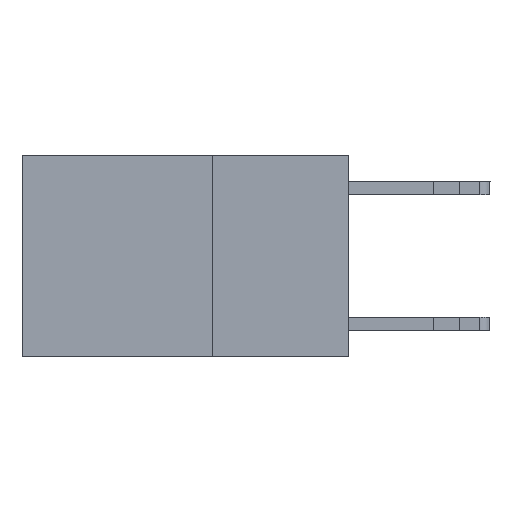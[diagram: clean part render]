
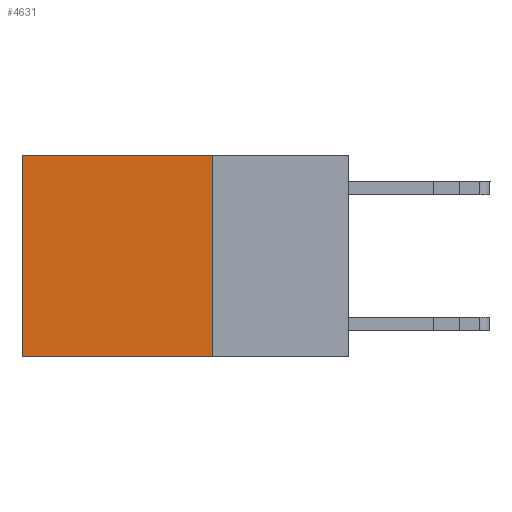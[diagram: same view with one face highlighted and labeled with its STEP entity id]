
A CAD part, left-side view. The second image highlights one B-rep face of the part: STEP entity #4631.
In plain terms, the highlighted planar face has unit normal (-1, 0, 0).
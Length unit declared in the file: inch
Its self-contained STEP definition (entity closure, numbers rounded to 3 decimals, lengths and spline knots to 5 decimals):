
#223 = DIRECTION ( 'NONE',  ( 0., 1., 0. ) ) ;
#496 = DIRECTION ( 'NONE',  ( 0., 1., 0. ) ) ;
#2611 = LINE ( 'NONE', #7251, #3424 ) ;
#2944 = CARTESIAN_POINT ( 'NONE',  ( 0.2625, 0.6, -0.37 ) ) ;
#3009 = ORIENTED_EDGE ( 'NONE', *, *, #6220, .T. ) ;
#3424 = VECTOR ( 'NONE', #496, 39.37008 ) ;
#4271 = DIRECTION ( 'NONE',  ( 1., 0., 0. ) ) ;
#4631 = ADVANCED_FACE ( 'NONE', ( #14182 ), #12147, .F. ) ;
#5284 = EDGE_CURVE ( 'NONE', #7028, #12721, #13727, .T. ) ;
#6003 = EDGE_CURVE ( 'NONE', #12983, #10503, #13409, .T. ) ;
#6211 = CARTESIAN_POINT ( 'NONE',  ( 0.2625, 0.25, 0. ) ) ;
#6220 = EDGE_CURVE ( 'NONE', #7028, #12983, #2611, .T. ) ;
#6309 = ORIENTED_EDGE ( 'NONE', *, *, #7378, .F. ) ;
#6672 = CARTESIAN_POINT ( 'NONE',  ( 0.2625, 0.25, 0. ) ) ;
#6841 = LINE ( 'NONE', #9230, #11049 ) ;
#7028 = VERTEX_POINT ( 'NONE', #9510 ) ;
#7251 = CARTESIAN_POINT ( 'NONE',  ( 0.2625, 0.25, 0. ) ) ;
#7378 = EDGE_CURVE ( 'NONE', #12721, #10503, #6841, .T. ) ;
#7656 = AXIS2_PLACEMENT_3D ( 'NONE', #6672, #4271, #12001 ) ;
#8067 = DIRECTION ( 'NONE',  ( 0., 0., -1. ) ) ;
#8513 = VECTOR ( 'NONE', #8067, 39.37008 ) ;
#8750 = ORIENTED_EDGE ( 'NONE', *, *, #5284, .F. ) ;
#9230 = CARTESIAN_POINT ( 'NONE',  ( 0.2625, 0.25, -0.37 ) ) ;
#9385 = DIRECTION ( 'NONE',  ( 0., 0., -1. ) ) ;
#9450 = EDGE_LOOP ( 'NONE', ( #12796, #6309, #8750, #3009 ) ) ;
#9510 = CARTESIAN_POINT ( 'NONE',  ( 0.2625, 0.25, 0. ) ) ;
#10503 = VERTEX_POINT ( 'NONE', #2944 ) ;
#10700 = CARTESIAN_POINT ( 'NONE',  ( 0.2625, 0.25, -0.37 ) ) ;
#11049 = VECTOR ( 'NONE', #223, 39.37008 ) ;
#12001 = DIRECTION ( 'NONE',  ( 0., 0., -1. ) ) ;
#12147 = PLANE ( 'NONE',  #7656 ) ;
#12241 = CARTESIAN_POINT ( 'NONE',  ( 0.2625, 0.6, 0. ) ) ;
#12401 = VECTOR ( 'NONE', #9385, 39.37008 ) ;
#12485 = CARTESIAN_POINT ( 'NONE',  ( 0.2625, 0.6, 0. ) ) ;
#12721 = VERTEX_POINT ( 'NONE', #10700 ) ;
#12796 = ORIENTED_EDGE ( 'NONE', *, *, #6003, .T. ) ;
#12983 = VERTEX_POINT ( 'NONE', #12485 ) ;
#13409 = LINE ( 'NONE', #12241, #8513 ) ;
#13727 = LINE ( 'NONE', #6211, #12401 ) ;
#14182 = FACE_OUTER_BOUND ( 'NONE', #9450, .T. ) ;
